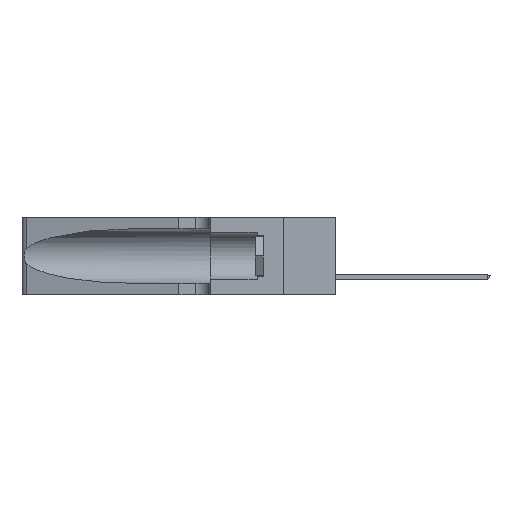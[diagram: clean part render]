
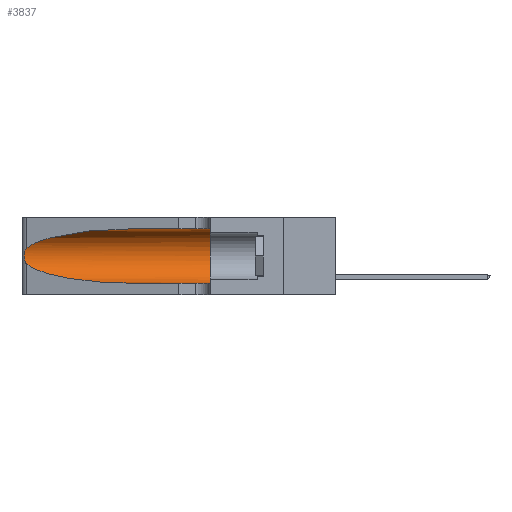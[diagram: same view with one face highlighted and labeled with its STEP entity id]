
A CAD part, left-side view. The second image highlights one B-rep face of the part: STEP entity #3837.
In plain terms, the highlighted cylindrical face has radius 3.308 mm (diameter 6.617 mm), a partial arc.
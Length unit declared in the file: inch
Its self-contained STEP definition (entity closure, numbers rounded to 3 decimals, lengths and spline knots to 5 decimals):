
#763 = ORIENTED_EDGE ( 'NONE', *, *, #26207, .T. ) ;
#780 = CARTESIAN_POINT ( 'NONE',  ( 0.25487, 1.22718, 0.22369 ) ) ;
#838 = VERTEX_POINT ( 'NONE', #2169 ) ;
#1606 = CARTESIAN_POINT ( 'NONE',  ( 0.1305, 1.61858, 0.31525 ) ) ;
#2169 = CARTESIAN_POINT ( 'NONE',  ( 0.1305, 0.72297, 0.05475 ) ) ;
#3837 = ADVANCED_FACE ( 'NONE', ( #6180 ), #30383, .F. ) ;
#4153 = CARTESIAN_POINT ( 'NONE',  ( 0.1305, 0.72297, 0.31525 ) ) ;
#4383 = CARTESIAN_POINT ( 'NONE',  ( 0.25487, 1.22718, 0.14631 ) ) ;
#6180 = FACE_OUTER_BOUND ( 'NONE', #24104, .T. ) ;
#6422 = CARTESIAN_POINT ( 'NONE',  ( 0.1305, 0.72297, 0.05475 ) ) ;
#7016 = CARTESIAN_POINT ( 'NONE',  ( 0.1305, 1.61858, 0.05475 ) ) ;
#7018 = CARTESIAN_POINT ( 'NONE',  ( 0.1305, 0.72297, 0.31525 ) ) ;
#9043 = VERTEX_POINT ( 'NONE', #33204 ) ;
#9556 = CARTESIAN_POINT ( 'NONE',  ( 0.1305, 0.35, 0.05475 ) ) ;
#11209 = CARTESIAN_POINT ( 'NONE',  ( 0.2373, 1.15595, 0.28018 ) ) ;
#11434 = CARTESIAN_POINT ( 'NONE',  ( 0.26075, 1.23896, 0.178 ) ) ;
#11582 = CARTESIAN_POINT ( 'NONE',  ( 0.26018, 1.23835, 0.19895 ) ) ;
#13463 = VECTOR ( 'NONE', #24575, 39.37008 ) ;
#13596 = ORIENTED_EDGE ( 'NONE', *, *, #24367, .T. ) ;
#14981 = CARTESIAN_POINT ( 'NONE',  ( 0.1305, 1.61858, 0.185 ) ) ;
#15087 = DIRECTION ( 'NONE',  ( 0., 1., 0. ) ) ;
#16851 = VECTOR ( 'NONE', #34117, 39.37008 ) ;
#18916 = CARTESIAN_POINT ( 'NONE',  ( 0.25787, 1.23484, 0.2124 ) ) ;
#19167 = EDGE_CURVE ( 'NONE', #20702, #9043, #40278, .T. ) ;
#19549 = AXIS2_PLACEMENT_3D ( 'NONE', #14981, #26090, #32663 ) ;
#20702 = VERTEX_POINT ( 'NONE', #7018 ) ;
#20734 = EDGE_CURVE ( 'NONE', #36302, #27410, #39001, .T. ) ;
#20929 = VERTEX_POINT ( 'NONE', #27141 ) ;
#21843 = CARTESIAN_POINT ( 'NONE',  ( 0.25854, 1.2359, 0.20912 ) ) ;
#23787 = CARTESIAN_POINT ( 'NONE',  ( 0.2373, 1.15595, 0.08982 ) ) ;
#24104 = EDGE_LOOP ( 'NONE', ( #30826, #26772, #763, #13596, #33976, #32169 ) ) ;
#24367 = EDGE_CURVE ( 'NONE', #838, #27410, #24390, .T. ) ;
#24390 = LINE ( 'NONE', #7016, #13463 ) ;
#24429 = AXIS2_PLACEMENT_3D ( 'NONE', #26027, #15087, #29240 ) ;
#24575 = DIRECTION ( 'NONE',  ( 0., -1., 0. ) ) ;
#26027 = CARTESIAN_POINT ( 'NONE',  ( 0.1305, 0.35, 0.185 ) ) ;
#26090 = DIRECTION ( 'NONE',  ( 0., -1., 0. ) ) ;
#26207 = EDGE_CURVE ( 'NONE', #20929, #838, #43628, .T. ) ;
#26545 = CARTESIAN_POINT ( 'NONE',  ( 0.25487, 1.22718, 0.14631 ) ) ;
#26772 = ORIENTED_EDGE ( 'NONE', *, *, #41591, .T. ) ;
#27141 = CARTESIAN_POINT ( 'NONE',  ( 0.25487, 1.22718, 0.14631 ) ) ;
#27410 = VERTEX_POINT ( 'NONE', #9556 ) ;
#28712 = CARTESIAN_POINT ( 'NONE',  ( 0.18966, 0.96281, 0.31525 ) ) ;
#29075 = CARTESIAN_POINT ( 'NONE',  ( 0.26017, 1.23833, 0.17102 ) ) ;
#29240 = DIRECTION ( 'NONE',  ( 0., 0., 1. ) ) ;
#30383 = CYLINDRICAL_SURFACE ( 'NONE', #19549, 0.13025 ) ;
#30826 = ORIENTED_EDGE ( 'NONE', *, *, #19167, .T. ) ;
#31046 = B_SPLINE_CURVE_WITH_KNOTS ( 'NONE', 3,
 ( #43282, #36259, #36425, #18916, #21843, #11582, #36104, #11434, #29075, #39465, #32769, #39780, #39623, #4383 ),
 .UNSPECIFIED., .F., .F.,
 ( 4, 2, 2, 2, 2, 2, 4 ),
 ( 0., 0.00027, 0.00053, 0.00107, 0.0016, 0.00187, 0.00214 ),
 .UNSPECIFIED. ) ;
#32169 = ORIENTED_EDGE ( 'NONE', *, *, #34775, .F. ) ;
#32663 = DIRECTION ( 'NONE',  ( 0., 0., -1. ) ) ;
#32769 = CARTESIAN_POINT ( 'NONE',  ( 0.25789, 1.23486, 0.15765 ) ) ;
#33204 = CARTESIAN_POINT ( 'NONE',  ( 0.25487, 1.22718, 0.22369 ) ) ;
#33976 = ORIENTED_EDGE ( 'NONE', *, *, #20734, .F. ) ;
#34117 = DIRECTION ( 'NONE',  ( 0., -1., 0. ) ) ;
#34775 = EDGE_CURVE ( 'NONE', #20702, #36302, #35491, .T. ) ;
#35491 = LINE ( 'NONE', #1606, #16851 ) ;
#36104 = CARTESIAN_POINT ( 'NONE',  ( 0.26075, 1.23896, 0.19203 ) ) ;
#36259 = CARTESIAN_POINT ( 'NONE',  ( 0.25555, 1.22994, 0.2215 ) ) ;
#36302 = VERTEX_POINT ( 'NONE', #38859 ) ;
#36425 = CARTESIAN_POINT ( 'NONE',  ( 0.25639, 1.23184, 0.21858 ) ) ;
#38859 = CARTESIAN_POINT ( 'NONE',  ( 0.1305, 0.35, 0.31525 ) ) ;
#39001 = CIRCLE ( 'NONE', #24429, 0.13025 ) ;
#39465 = CARTESIAN_POINT ( 'NONE',  ( 0.25856, 1.23593, 0.16098 ) ) ;
#39623 = CARTESIAN_POINT ( 'NONE',  ( 0.25555, 1.22993, 0.14849 ) ) ;
#39780 = CARTESIAN_POINT ( 'NONE',  ( 0.25639, 1.23186, 0.15144 ) ) ;
#40278 =( BOUNDED_CURVE ( )  B_SPLINE_CURVE ( 3, ( #4153, #28712, #11209, #780 ),
 .UNSPECIFIED., .F., .F. ) 
 B_SPLINE_CURVE_WITH_KNOTS ( ( 4, 4 ),
 ( 1.5708, 2.84003 ),
 .UNSPECIFIED. ) 
 CURVE ( )  GEOMETRIC_REPRESENTATION_ITEM ( )  RATIONAL_B_SPLINE_CURVE ( ( 1., 0.87, 0.87, 1. ) ) 
 REPRESENTATION_ITEM ( '' )  );
#41367 = CARTESIAN_POINT ( 'NONE',  ( 0.18966, 0.96281, 0.05475 ) ) ;
#41591 = EDGE_CURVE ( 'NONE', #9043, #20929, #31046, .T. ) ;
#43282 = CARTESIAN_POINT ( 'NONE',  ( 0.25487, 1.22718, 0.22369 ) ) ;
#43628 =( BOUNDED_CURVE ( )  B_SPLINE_CURVE ( 3, ( #26545, #23787, #41367, #6422 ),
 .UNSPECIFIED., .F., .F. ) 
 B_SPLINE_CURVE_WITH_KNOTS ( ( 4, 4 ),
 ( 3.44316, 4.71239 ),
 .UNSPECIFIED. ) 
 CURVE ( )  GEOMETRIC_REPRESENTATION_ITEM ( )  RATIONAL_B_SPLINE_CURVE ( ( 1., 0.87, 0.87, 1. ) ) 
 REPRESENTATION_ITEM ( '' )  );
